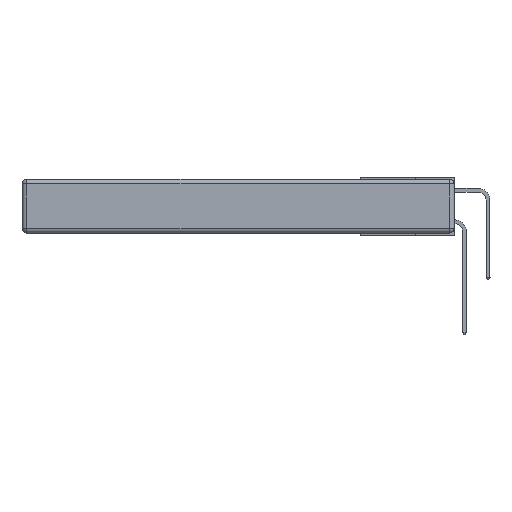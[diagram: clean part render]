
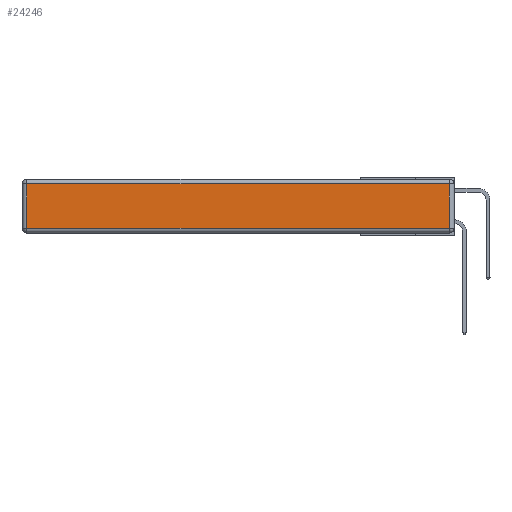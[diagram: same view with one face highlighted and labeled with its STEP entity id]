
A CAD part, left-side view. The second image highlights one B-rep face of the part: STEP entity #24246.
In plain terms, the highlighted planar face has unit normal (-1, 0, 0).
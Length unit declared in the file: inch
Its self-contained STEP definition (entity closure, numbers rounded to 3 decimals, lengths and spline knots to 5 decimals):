
#688 = DIRECTION ( 'NONE',  ( 0., 0., 1. ) ) ;
#863 = VERTEX_POINT ( 'NONE', #17508 ) ;
#1633 = CARTESIAN_POINT ( 'NONE',  ( 0., 2.72, -0.03 ) ) ;
#1869 = AXIS2_PLACEMENT_3D ( 'NONE', #6433, #3565, #688 ) ;
#3184 = ORIENTED_EDGE ( 'NONE', *, *, #17512, .T. ) ;
#3565 = DIRECTION ( 'NONE',  ( -1., 0., 0. ) ) ;
#4896 = VECTOR ( 'NONE', #14919, 39.37008 ) ;
#5196 = LINE ( 'NONE', #36690, #33933 ) ;
#5354 = ORIENTED_EDGE ( 'NONE', *, *, #34472, .T. ) ;
#6433 = CARTESIAN_POINT ( 'NONE',  ( 0., 0., -0.343 ) ) ;
#6474 = DIRECTION ( 'NONE',  ( 0., 1., 0. ) ) ;
#6918 = CARTESIAN_POINT ( 'NONE',  ( 0., 2.72, -0.343 ) ) ;
#7533 = VECTOR ( 'NONE', #26662, 39.37008 ) ;
#11393 = VERTEX_POINT ( 'NONE', #16555 ) ;
#11994 = FACE_OUTER_BOUND ( 'NONE', #13386, .T. ) ;
#12271 = EDGE_CURVE ( 'NONE', #11393, #863, #5196, .T. ) ;
#12478 = PLANE ( 'NONE',  #1869 ) ;
#12733 = VERTEX_POINT ( 'NONE', #26636 ) ;
#13386 = EDGE_LOOP ( 'NONE', ( #23943, #36338, #5354, #3184 ) ) ;
#14097 = DIRECTION ( 'NONE',  ( 0., 0., 1. ) ) ;
#14550 = CARTESIAN_POINT ( 'NONE',  ( 0., 0., -0.313 ) ) ;
#14919 = DIRECTION ( 'NONE',  ( 0., -1., 0. ) ) ;
#16555 = CARTESIAN_POINT ( 'NONE',  ( 0., 0.03, -0.313 ) ) ;
#17372 = VECTOR ( 'NONE', #6474, 39.37008 ) ;
#17508 = CARTESIAN_POINT ( 'NONE',  ( 0., 0.03, -0.03 ) ) ;
#17512 = EDGE_CURVE ( 'NONE', #31976, #12733, #26431, .T. ) ;
#23943 = ORIENTED_EDGE ( 'NONE', *, *, #26862, .T. ) ;
#24246 = ADVANCED_FACE ( 'NONE', ( #11994 ), #12478, .T. ) ;
#25947 = LINE ( 'NONE', #32224, #17372 ) ;
#26431 = LINE ( 'NONE', #6918, #7533 ) ;
#26636 = CARTESIAN_POINT ( 'NONE',  ( 0., 2.72, -0.313 ) ) ;
#26662 = DIRECTION ( 'NONE',  ( 0., 0., -1. ) ) ;
#26862 = EDGE_CURVE ( 'NONE', #12733, #11393, #27848, .T. ) ;
#27848 = LINE ( 'NONE', #14550, #4896 ) ;
#31976 = VERTEX_POINT ( 'NONE', #1633 ) ;
#32224 = CARTESIAN_POINT ( 'NONE',  ( 0., 2.75, -0.03 ) ) ;
#33933 = VECTOR ( 'NONE', #14097, 39.37008 ) ;
#34472 = EDGE_CURVE ( 'NONE', #863, #31976, #25947, .T. ) ;
#36338 = ORIENTED_EDGE ( 'NONE', *, *, #12271, .T. ) ;
#36690 = CARTESIAN_POINT ( 'NONE',  ( 0., 0.03, -0.343 ) ) ;
